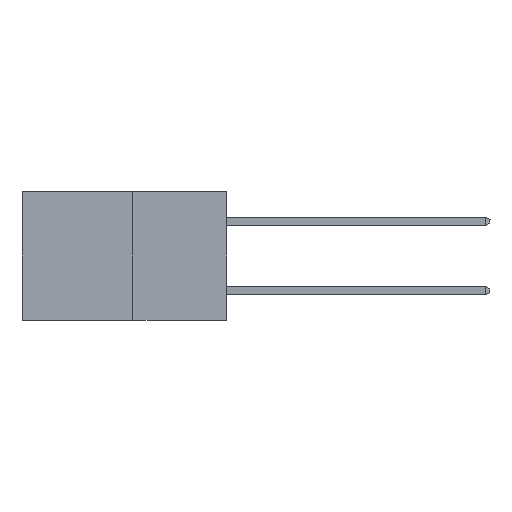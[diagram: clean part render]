
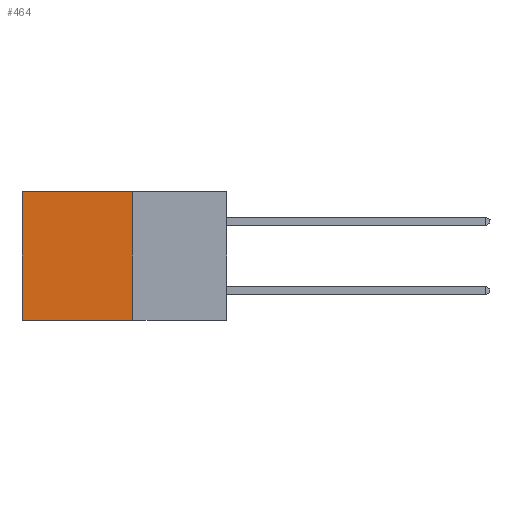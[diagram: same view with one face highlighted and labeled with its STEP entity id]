
A CAD part, left-side view. The second image highlights one B-rep face of the part: STEP entity #464.
In plain terms, the highlighted planar face has unit normal (-1, 0, 0).
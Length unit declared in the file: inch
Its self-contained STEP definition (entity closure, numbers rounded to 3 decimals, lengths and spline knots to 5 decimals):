
#61 = CARTESIAN_POINT ( 'NONE',  ( 0.277, 0.59, -0.37 ) ) ;
#177 = ORIENTED_EDGE ( 'NONE', *, *, #8577, .T. ) ;
#298 = CARTESIAN_POINT ( 'NONE',  ( 0.277, 0.59, 0. ) ) ;
#464 = ADVANCED_FACE ( 'NONE', ( #2904 ), #3600, .F. ) ;
#590 = VECTOR ( 'NONE', #11742, 39.37008 ) ;
#1051 = EDGE_CURVE ( 'NONE', #1112, #3405, #11143, .T. ) ;
#1112 = VERTEX_POINT ( 'NONE', #6596 ) ;
#1182 = LINE ( 'NONE', #8951, #10981 ) ;
#1276 = EDGE_CURVE ( 'NONE', #10275, #9847, #1182, .T. ) ;
#1706 = EDGE_CURVE ( 'NONE', #3405, #9847, #3472, .T. ) ;
#2548 = CARTESIAN_POINT ( 'NONE',  ( 0.277, 0.27, -0.37 ) ) ;
#2904 = FACE_OUTER_BOUND ( 'NONE', #4322, .T. ) ;
#3006 = DIRECTION ( 'NONE',  ( 0., 0., -1. ) ) ;
#3010 = ORIENTED_EDGE ( 'NONE', *, *, #1276, .T. ) ;
#3216 = CARTESIAN_POINT ( 'NONE',  ( 0.277, 0.27, -0.37 ) ) ;
#3362 = AXIS2_PLACEMENT_3D ( 'NONE', #3216, #9948, #3006 ) ;
#3405 = VERTEX_POINT ( 'NONE', #2548 ) ;
#3472 = LINE ( 'NONE', #7133, #590 ) ;
#3600 = PLANE ( 'NONE',  #3362 ) ;
#3788 = DIRECTION ( 'NONE',  ( 0., 0., -1. ) ) ;
#4322 = EDGE_LOOP ( 'NONE', ( #3010, #7392, #11948, #177 ) ) ;
#5203 = CARTESIAN_POINT ( 'NONE',  ( 0.277, 0.27, -0.37 ) ) ;
#6596 = CARTESIAN_POINT ( 'NONE',  ( 0.277, 0.27, 0. ) ) ;
#6987 = VECTOR ( 'NONE', #11250, 39.37008 ) ;
#7133 = CARTESIAN_POINT ( 'NONE',  ( 0.277, 0.27, -0.37 ) ) ;
#7392 = ORIENTED_EDGE ( 'NONE', *, *, #1706, .F. ) ;
#7595 = DIRECTION ( 'NONE',  ( 0., 0., -1. ) ) ;
#8577 = EDGE_CURVE ( 'NONE', #1112, #10275, #12126, .T. ) ;
#8586 = VECTOR ( 'NONE', #3788, 39.37008 ) ;
#8951 = CARTESIAN_POINT ( 'NONE',  ( 0.277, 0.59, -0.37 ) ) ;
#9284 = CARTESIAN_POINT ( 'NONE',  ( 0.277, 0.27, 0. ) ) ;
#9847 = VERTEX_POINT ( 'NONE', #61 ) ;
#9948 = DIRECTION ( 'NONE',  ( 1., 0., 0. ) ) ;
#10275 = VERTEX_POINT ( 'NONE', #298 ) ;
#10981 = VECTOR ( 'NONE', #7595, 39.37008 ) ;
#11143 = LINE ( 'NONE', #5203, #8586 ) ;
#11250 = DIRECTION ( 'NONE',  ( 0., 1., 0. ) ) ;
#11742 = DIRECTION ( 'NONE',  ( 0., 1., 0. ) ) ;
#11948 = ORIENTED_EDGE ( 'NONE', *, *, #1051, .F. ) ;
#12126 = LINE ( 'NONE', #9284, #6987 ) ;
